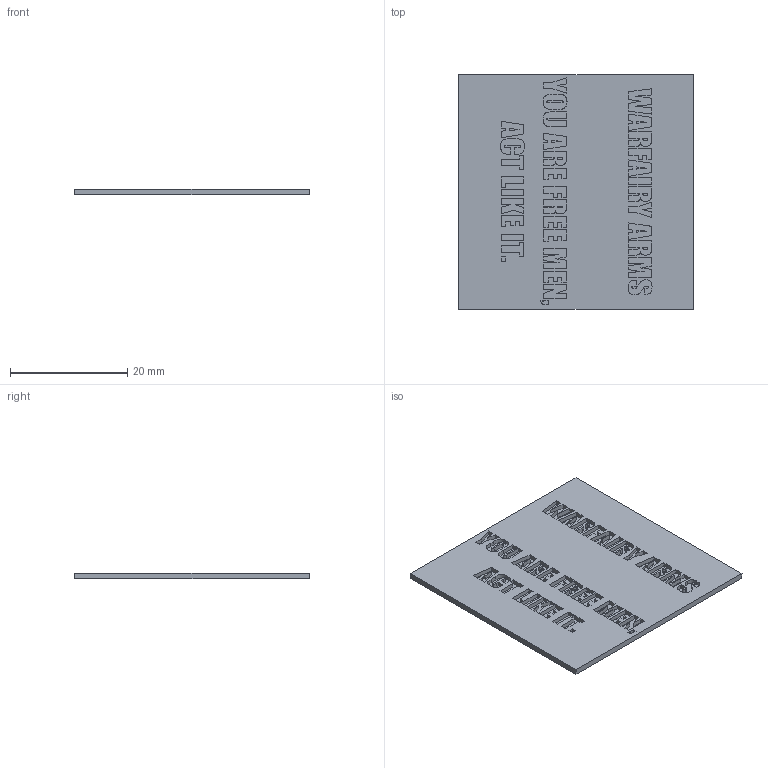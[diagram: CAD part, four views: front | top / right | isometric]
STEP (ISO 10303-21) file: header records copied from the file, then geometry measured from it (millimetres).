
FILE_DESCRIPTION (( 'STEP AP214' ), '1' );
FILE_NAME ('WarFairy.STEP', '2013-09-01T16:53:01', ( 'Asher' ), ( '' ), 'SwSTEP 2.0', 'SolidWorks 2013', '' );
FILE_SCHEMA (( 'AUTOMOTIVE_DESIGN' ));
Length unit declared in the file: millimetre
Products named in the file (1): WarFairy
Bounding box: 40 x 40 x 1 mm (x, y, z)
Volume: 1413.9 mm3; surface area: 3791.2 mm2
Topology: 1 solids, 1 shells, 449 faces, 1200 edges, 800 vertices
Faces by surface type: plane 361, bspline 88
Entity records: 18704 total; most frequent: CARTESIAN_POINT 8042, ORIENTED_EDGE 2400, DIRECTION 1748, EDGE_CURVE 1200, LINE 1024, VECTOR 1024, VERTEX_POINT 800, EDGE_LOOP 496
